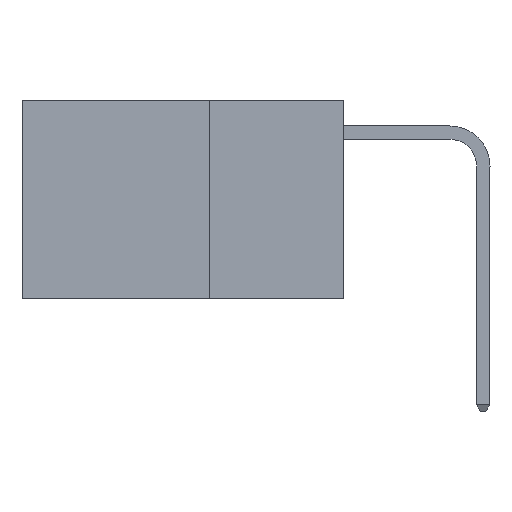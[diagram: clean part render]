
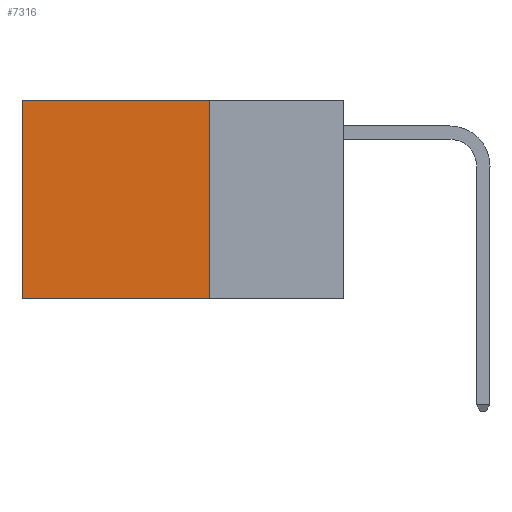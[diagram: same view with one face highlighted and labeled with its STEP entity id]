
A CAD part, left-side view. The second image highlights one B-rep face of the part: STEP entity #7316.
In plain terms, the highlighted planar face has unit normal (-1, 0, 0).
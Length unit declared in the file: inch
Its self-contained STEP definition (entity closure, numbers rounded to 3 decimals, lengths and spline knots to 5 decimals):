
#432 = LINE ( 'NONE', #6408, #6243 ) ;
#1475 = VECTOR ( 'NONE', #11931, 39.37008 ) ;
#1634 = EDGE_CURVE ( 'NONE', #9176, #9035, #1853, .T. ) ;
#1853 = LINE ( 'NONE', #9628, #1475 ) ;
#1915 = VERTEX_POINT ( 'NONE', #5652 ) ;
#2066 = ORIENTED_EDGE ( 'NONE', *, *, #14535, .F. ) ;
#2824 = PLANE ( 'NONE',  #4556 ) ;
#3003 = CARTESIAN_POINT ( 'NONE',  ( 0.2625, 0.6, -0.37 ) ) ;
#3013 = DIRECTION ( 'NONE',  ( 0., 0., -1. ) ) ;
#4411 = VECTOR ( 'NONE', #12773, 39.37008 ) ;
#4556 = AXIS2_PLACEMENT_3D ( 'NONE', #12026, #5082, #13201 ) ;
#5082 = DIRECTION ( 'NONE',  ( 1., 0., 0. ) ) ;
#5316 = VERTEX_POINT ( 'NONE', #3003 ) ;
#5652 = CARTESIAN_POINT ( 'NONE',  ( 0.2625, 0.25, -0.37 ) ) ;
#6243 = VECTOR ( 'NONE', #12193, 39.37008 ) ;
#6408 = CARTESIAN_POINT ( 'NONE',  ( 0.2625, 0.25, -0.37 ) ) ;
#6419 = EDGE_CURVE ( 'NONE', #9035, #5316, #10191, .T. ) ;
#7316 = ADVANCED_FACE ( 'NONE', ( #9787 ), #2824, .F. ) ;
#8522 = CARTESIAN_POINT ( 'NONE',  ( 0.2625, 0.6, 0. ) ) ;
#8709 = VECTOR ( 'NONE', #3013, 39.37008 ) ;
#8717 = CARTESIAN_POINT ( 'NONE',  ( 0.2625, 0.25, 0. ) ) ;
#9035 = VERTEX_POINT ( 'NONE', #8522 ) ;
#9176 = VERTEX_POINT ( 'NONE', #11157 ) ;
#9438 = LINE ( 'NONE', #8717, #8709 ) ;
#9628 = CARTESIAN_POINT ( 'NONE',  ( 0.2625, 0.25, 0. ) ) ;
#9787 = FACE_OUTER_BOUND ( 'NONE', #11717, .T. ) ;
#10191 = LINE ( 'NONE', #10431, #4411 ) ;
#10431 = CARTESIAN_POINT ( 'NONE',  ( 0.2625, 0.6, 0. ) ) ;
#11157 = CARTESIAN_POINT ( 'NONE',  ( 0.2625, 0.25, 0. ) ) ;
#11539 = EDGE_CURVE ( 'NONE', #9176, #1915, #9438, .T. ) ;
#11717 = EDGE_LOOP ( 'NONE', ( #12487, #2066, #13608, #11754 ) ) ;
#11754 = ORIENTED_EDGE ( 'NONE', *, *, #1634, .T. ) ;
#11931 = DIRECTION ( 'NONE',  ( 0., 1., 0. ) ) ;
#12026 = CARTESIAN_POINT ( 'NONE',  ( 0.2625, 0.25, 0. ) ) ;
#12193 = DIRECTION ( 'NONE',  ( 0., 1., 0. ) ) ;
#12487 = ORIENTED_EDGE ( 'NONE', *, *, #6419, .T. ) ;
#12773 = DIRECTION ( 'NONE',  ( 0., 0., -1. ) ) ;
#13201 = DIRECTION ( 'NONE',  ( 0., 0., -1. ) ) ;
#13608 = ORIENTED_EDGE ( 'NONE', *, *, #11539, .F. ) ;
#14535 = EDGE_CURVE ( 'NONE', #1915, #5316, #432, .T. ) ;
